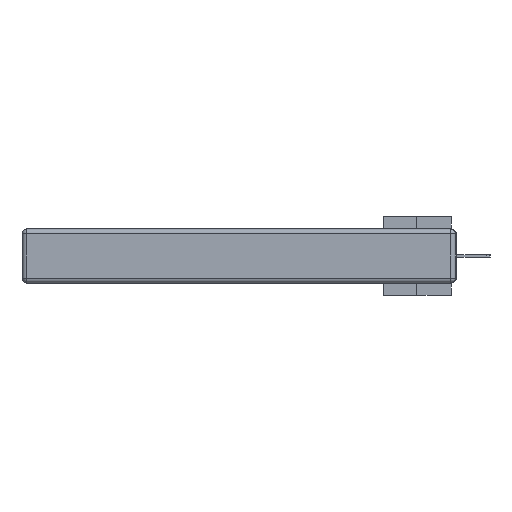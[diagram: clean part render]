
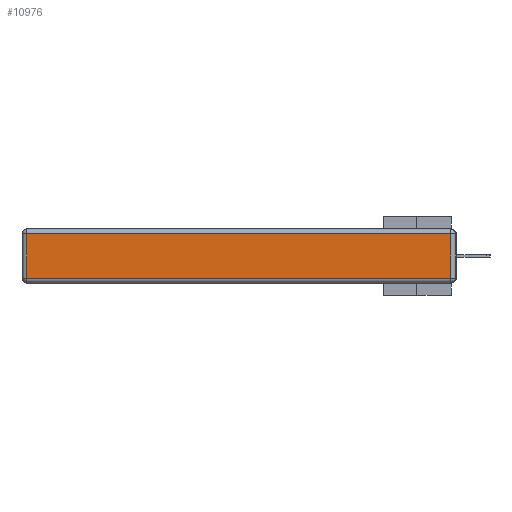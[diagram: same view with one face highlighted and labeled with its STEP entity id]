
A CAD part, left-side view. The second image highlights one B-rep face of the part: STEP entity #10976.
In plain terms, the highlighted planar face has unit normal (-1, 0, 0).
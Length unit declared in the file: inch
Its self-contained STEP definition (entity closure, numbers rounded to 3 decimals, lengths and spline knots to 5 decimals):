
#822 = EDGE_CURVE ( 'NONE', #39731, #32577, #18424, .T. ) ;
#847 = LINE ( 'NONE', #33485, #36456 ) ;
#3456 = DIRECTION ( 'NONE',  ( -1., 0., 0. ) ) ;
#4579 = VECTOR ( 'NONE', #14390, 39.37008 ) ;
#4681 = ORIENTED_EDGE ( 'NONE', *, *, #22377, .T. ) ;
#6442 = ORIENTED_EDGE ( 'NONE', *, *, #822, .T. ) ;
#7329 = EDGE_LOOP ( 'NONE', ( #4681, #40292, #14476, #6442 ) ) ;
#10915 = DIRECTION ( 'NONE',  ( 0., 0., 1. ) ) ;
#10976 = ADVANCED_FACE ( 'NONE', ( #19771 ), #29739, .T. ) ;
#12703 = EDGE_CURVE ( 'NONE', #37207, #39731, #847, .T. ) ;
#14071 = CARTESIAN_POINT ( 'NONE',  ( 0., 0.03, -0.343 ) ) ;
#14390 = DIRECTION ( 'NONE',  ( 0., 0., -1. ) ) ;
#14476 = ORIENTED_EDGE ( 'NONE', *, *, #12703, .T. ) ;
#16138 = EDGE_CURVE ( 'NONE', #19826, #37207, #39951, .T. ) ;
#16183 = CARTESIAN_POINT ( 'NONE',  ( 0., 2.72, -0.313 ) ) ;
#18424 = LINE ( 'NONE', #30775, #4579 ) ;
#19771 = FACE_OUTER_BOUND ( 'NONE', #7329, .T. ) ;
#19826 = VERTEX_POINT ( 'NONE', #34875 ) ;
#19905 = CARTESIAN_POINT ( 'NONE',  ( 0., 0.03, -0.03 ) ) ;
#21382 = LINE ( 'NONE', #27759, #22023 ) ;
#22023 = VECTOR ( 'NONE', #28579, 39.37008 ) ;
#22377 = EDGE_CURVE ( 'NONE', #32577, #19826, #21382, .T. ) ;
#27491 = AXIS2_PLACEMENT_3D ( 'NONE', #32706, #3456, #35680 ) ;
#27759 = CARTESIAN_POINT ( 'NONE',  ( 0., 0., -0.313 ) ) ;
#28579 = DIRECTION ( 'NONE',  ( 0., -1., 0. ) ) ;
#29739 = PLANE ( 'NONE',  #27491 ) ;
#30097 = DIRECTION ( 'NONE',  ( 0., 1., 0. ) ) ;
#30775 = CARTESIAN_POINT ( 'NONE',  ( 0., 2.72, -0.343 ) ) ;
#32577 = VERTEX_POINT ( 'NONE', #16183 ) ;
#32706 = CARTESIAN_POINT ( 'NONE',  ( 0., 0., -0.343 ) ) ;
#33036 = VECTOR ( 'NONE', #10915, 39.37008 ) ;
#33485 = CARTESIAN_POINT ( 'NONE',  ( 0., 2.75, -0.03 ) ) ;
#34780 = CARTESIAN_POINT ( 'NONE',  ( 0., 2.72, -0.03 ) ) ;
#34875 = CARTESIAN_POINT ( 'NONE',  ( 0., 0.03, -0.313 ) ) ;
#35680 = DIRECTION ( 'NONE',  ( 0., 0., 1. ) ) ;
#36456 = VECTOR ( 'NONE', #30097, 39.37008 ) ;
#37207 = VERTEX_POINT ( 'NONE', #19905 ) ;
#39731 = VERTEX_POINT ( 'NONE', #34780 ) ;
#39951 = LINE ( 'NONE', #14071, #33036 ) ;
#40292 = ORIENTED_EDGE ( 'NONE', *, *, #16138, .T. ) ;
